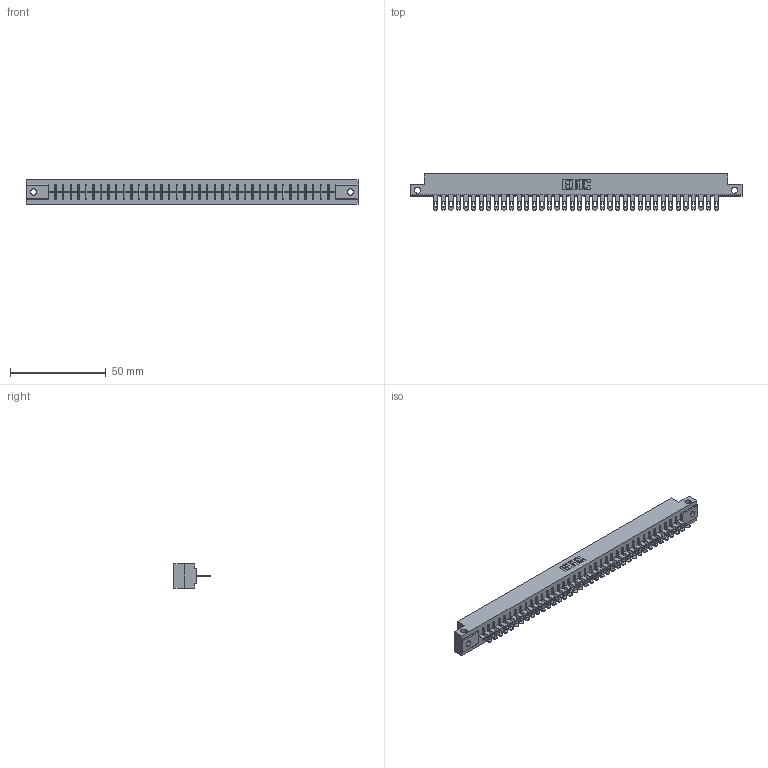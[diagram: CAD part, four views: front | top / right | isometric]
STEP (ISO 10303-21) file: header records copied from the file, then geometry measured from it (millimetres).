
FILE_DESCRIPTION (( 'STEP AP203' ), '1' );
FILE_NAME ('316-038-400-112.STEP', '2020-09-23T05:45:18', ( '' ), ( '' ), 'SwSTEP 2.0', 'SolidWorks 2020', '' );
FILE_SCHEMA (( 'CONFIG_CONTROL_DESIGN' ));
Length unit declared in the file: inch
Products named in the file (3): 316-038-400-112; 306 Part_.128 Dia; 306-290-001_100
Assembly tree (39 placements, depth 2):
  316-038-400-112
    306 Part_.128 Dia
    306-290-001_100  x38
Bounding box: 173.58 x 18.87 x 12.7 mm (x, y, z)
Volume: 19087.6 mm3; surface area: 20240.2 mm2
Topology: 39 solids, 39 shells, 3016 faces, 8522 edges, 5472 vertices
Faces by surface type: plane 1968, cylinder 896, sphere 152
Entity records: 36525 total; most frequent: CARTESIAN_POINT 6181, ORIENTED_EDGE 6084, DIRECTION 6034, EDGE_CURVE 3042, VECTOR 2360, LINE 2360, VERTEX_POINT 1920, AXIS2_PLACEMENT_3D 1837
